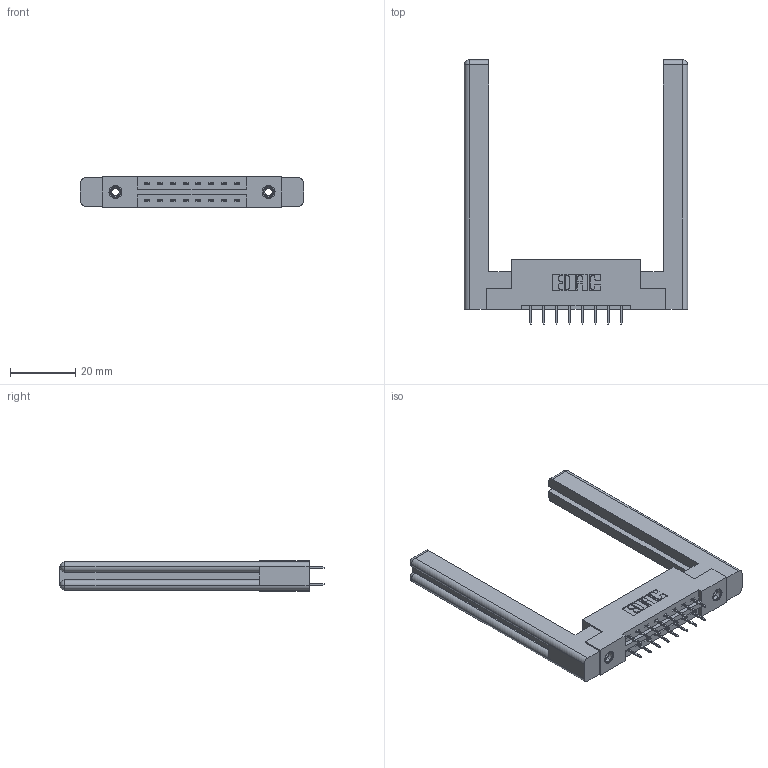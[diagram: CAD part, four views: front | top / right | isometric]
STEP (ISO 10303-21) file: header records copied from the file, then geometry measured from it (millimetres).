
FILE_DESCRIPTION (( 'STEP AP203' ), '1' );
FILE_NAME ('337-016-524-258.STEP', '2019-10-08T12:23:06', ( '' ), ( '' ), 'SwSTEP 2.0', 'SolidWorks 2016', '' );
FILE_SCHEMA (( 'CONFIG_CONTROL_DESIGN' ));
Length unit declared in the file: inch
Products named in the file (5): 345-250-001_345-250-001-102; 345-292-001_345-293-124; 337-016-524-258; 337 Part_Flush Mounting Lugs - 0.156 Dia-TI; 307-220-058
Assembly tree (21 placements, depth 2):
  337-016-524-258
    337 Part_Flush Mounting Lugs - 0.156 Dia-TI
    345-292-001_345-293-124  x16
    345-250-001_345-250-001-102  x2
    307-220-058  x2
Bounding box: 68.33 x 80.78 x 9.4 mm (x, y, z)
Volume: 13866.3 mm3; surface area: 12242.9 mm2
Topology: 21 solids, 21 shells, 1184 faces, 3305 edges, 2126 vertices
Faces by surface type: plane 858, cylinder 302, cone 12, torus 12
Entity records: 13308 total; most frequent: CARTESIAN_POINT 2277, ORIENTED_EDGE 2152, DIRECTION 2016, EDGE_CURVE 1076, LINE 904, VECTOR 904, VERTEX_POINT 706, AXIS2_PLACEMENT_3D 556
